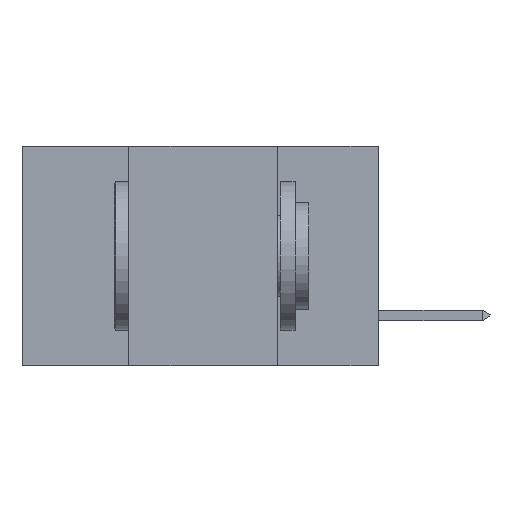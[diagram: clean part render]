
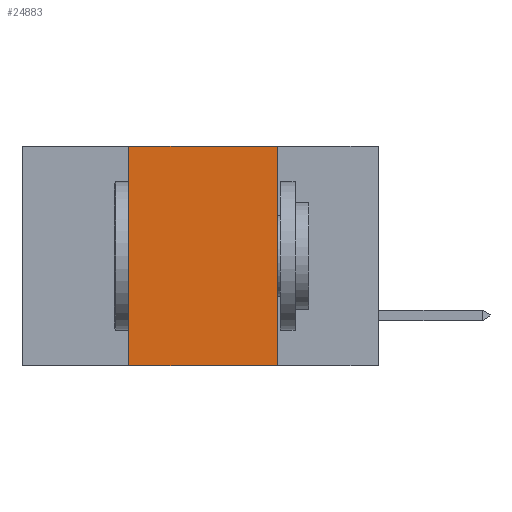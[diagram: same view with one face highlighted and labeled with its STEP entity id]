
A CAD part, left-side view. The second image highlights one B-rep face of the part: STEP entity #24883.
In plain terms, the highlighted planar face has unit normal (-1, 0, 0).
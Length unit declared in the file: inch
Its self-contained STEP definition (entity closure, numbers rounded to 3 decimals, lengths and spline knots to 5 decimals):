
#1511 = EDGE_CURVE ( 'NONE', #14208, #23334, #25507, .T. ) ;
#1814 = AXIS2_PLACEMENT_3D ( 'NONE', #6299, #20920, #16896 ) ;
#2424 = LINE ( 'NONE', #27152, #24577 ) ;
#2454 = FACE_OUTER_BOUND ( 'NONE', #10355, .T. ) ;
#2683 = VECTOR ( 'NONE', #9868, 39.37008 ) ;
#4520 = LINE ( 'NONE', #27809, #6196 ) ;
#6196 = VECTOR ( 'NONE', #21476, 39.37008 ) ;
#6299 = CARTESIAN_POINT ( 'NONE',  ( 0., 0.6, 0. ) ) ;
#8741 = CARTESIAN_POINT ( 'NONE',  ( 0., 0.42, -0.37 ) ) ;
#9117 = ORIENTED_EDGE ( 'NONE', *, *, #17898, .F. ) ;
#9280 = ORIENTED_EDGE ( 'NONE', *, *, #1511, .F. ) ;
#9868 = DIRECTION ( 'NONE',  ( 0., -1., 0. ) ) ;
#10049 = CARTESIAN_POINT ( 'NONE',  ( 0., 0.6, 0. ) ) ;
#10355 = EDGE_LOOP ( 'NONE', ( #9117, #9280, #17440, #26208 ) ) ;
#12201 = DIRECTION ( 'NONE',  ( 0., 0., -1. ) ) ;
#12692 = EDGE_CURVE ( 'NONE', #19032, #14208, #4520, .T. ) ;
#14208 = VERTEX_POINT ( 'NONE', #22071 ) ;
#14483 = CARTESIAN_POINT ( 'NONE',  ( 0., 0.17, 0. ) ) ;
#14515 = CARTESIAN_POINT ( 'NONE',  ( 0., 0.6, -0.37 ) ) ;
#16896 = DIRECTION ( 'NONE',  ( 0., 0., -1. ) ) ;
#16985 = PLANE ( 'NONE',  #1814 ) ;
#17440 = ORIENTED_EDGE ( 'NONE', *, *, #12692, .F. ) ;
#17898 = EDGE_CURVE ( 'NONE', #23334, #20427, #2424, .T. ) ;
#18099 = CARTESIAN_POINT ( 'NONE',  ( 0., 0.17, -0.37 ) ) ;
#18205 = EDGE_CURVE ( 'NONE', #19032, #20427, #26909, .T. ) ;
#19032 = VERTEX_POINT ( 'NONE', #8741 ) ;
#20427 = VERTEX_POINT ( 'NONE', #18099 ) ;
#20833 = VECTOR ( 'NONE', #22962, 39.37008 ) ;
#20920 = DIRECTION ( 'NONE',  ( 1., 0., 0. ) ) ;
#21476 = DIRECTION ( 'NONE',  ( 0., 0., 1. ) ) ;
#22071 = CARTESIAN_POINT ( 'NONE',  ( 0., 0.42, 0. ) ) ;
#22962 = DIRECTION ( 'NONE',  ( 0., -1., 0. ) ) ;
#23334 = VERTEX_POINT ( 'NONE', #14483 ) ;
#24577 = VECTOR ( 'NONE', #12201, 39.37008 ) ;
#24883 = ADVANCED_FACE ( 'NONE', ( #2454 ), #16985, .F. ) ;
#25507 = LINE ( 'NONE', #10049, #2683 ) ;
#26208 = ORIENTED_EDGE ( 'NONE', *, *, #18205, .T. ) ;
#26909 = LINE ( 'NONE', #14515, #20833 ) ;
#27152 = CARTESIAN_POINT ( 'NONE',  ( 0., 0.17, 0. ) ) ;
#27809 = CARTESIAN_POINT ( 'NONE',  ( 0., 0.42, 0. ) ) ;
